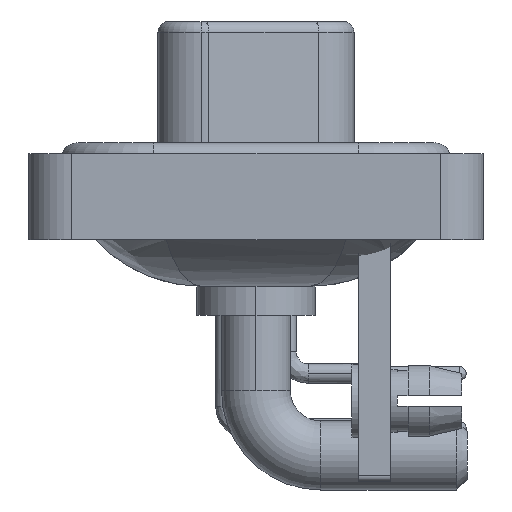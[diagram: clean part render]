
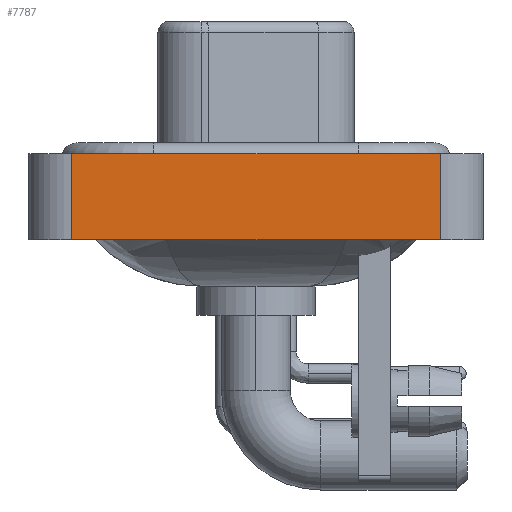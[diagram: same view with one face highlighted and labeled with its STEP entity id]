
A CAD part, left-side view. The second image highlights one B-rep face of the part: STEP entity #7787.
In plain terms, the highlighted planar face has unit normal (-1, 0, 0).
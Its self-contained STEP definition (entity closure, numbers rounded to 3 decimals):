
#1784 = LINE ( 'NONE', #29383, #1939 ) ;
#1939 = VECTOR ( 'NONE', #4165, 1000. ) ;
#3527 = AXIS2_PLACEMENT_3D ( 'NONE', #11396, #4631, #20578 ) ;
#4165 = DIRECTION ( 'NONE',  ( 0., -1., 0. ) ) ;
#4631 = DIRECTION ( 'NONE',  ( -1., 0., 0. ) ) ;
#5551 = DIRECTION ( 'NONE',  ( 0., 0., 1. ) ) ;
#6784 = LINE ( 'NONE', #25597, #21959 ) ;
#7787 = ADVANCED_FACE ( 'NONE', ( #13265 ), #15378, .T. ) ;
#8622 = VERTEX_POINT ( 'NONE', #23340 ) ;
#10127 = CARTESIAN_POINT ( 'NONE',  ( -7.35, -8.55, 0.4 ) ) ;
#11396 = CARTESIAN_POINT ( 'NONE',  ( -7.35, -8.55, -3.6 ) ) ;
#11677 = EDGE_CURVE ( 'NONE', #8622, #28525, #6784, .T. ) ;
#12551 = EDGE_CURVE ( 'NONE', #17456, #16141, #16973, .T. ) ;
#13265 = FACE_OUTER_BOUND ( 'NONE', #28422, .T. ) ;
#15378 = PLANE ( 'NONE',  #3527 ) ;
#15593 = CARTESIAN_POINT ( 'NONE',  ( -7.35, 8.55, 0.4 ) ) ;
#15943 = CARTESIAN_POINT ( 'NONE',  ( -7.35, -8.55, 0.4 ) ) ;
#16141 = VERTEX_POINT ( 'NONE', #10127 ) ;
#16240 = DIRECTION ( 'NONE',  ( 0., -1., 0. ) ) ;
#16973 = LINE ( 'NONE', #26164, #18151 ) ;
#17456 = VERTEX_POINT ( 'NONE', #23867 ) ;
#18151 = VECTOR ( 'NONE', #5551, 1000. ) ;
#19546 = VECTOR ( 'NONE', #16240, 1000. ) ;
#19998 = ORIENTED_EDGE ( 'NONE', *, *, #22440, .T. ) ;
#20578 = DIRECTION ( 'NONE',  ( 0., 0., 1. ) ) ;
#20625 = LINE ( 'NONE', #15943, #19546 ) ;
#20932 = DIRECTION ( 'NONE',  ( 0., 0., 1. ) ) ;
#21959 = VECTOR ( 'NONE', #20932, 1000. ) ;
#22440 = EDGE_CURVE ( 'NONE', #8622, #17456, #1784, .T. ) ;
#23340 = CARTESIAN_POINT ( 'NONE',  ( -7.35, 8.55, -3.6 ) ) ;
#23450 = ORIENTED_EDGE ( 'NONE', *, *, #11677, .F. ) ;
#23867 = CARTESIAN_POINT ( 'NONE',  ( -7.35, -8.55, -3.6 ) ) ;
#25261 = EDGE_CURVE ( 'NONE', #28525, #16141, #20625, .T. ) ;
#25597 = CARTESIAN_POINT ( 'NONE',  ( -7.35, 8.55, -3.6 ) ) ;
#26164 = CARTESIAN_POINT ( 'NONE',  ( -7.35, -8.55, -3.6 ) ) ;
#28422 = EDGE_LOOP ( 'NONE', ( #28997, #29266, #23450, #19998 ) ) ;
#28525 = VERTEX_POINT ( 'NONE', #15593 ) ;
#28997 = ORIENTED_EDGE ( 'NONE', *, *, #12551, .T. ) ;
#29266 = ORIENTED_EDGE ( 'NONE', *, *, #25261, .F. ) ;
#29383 = CARTESIAN_POINT ( 'NONE',  ( -7.35, -8.55, -3.6 ) ) ;
